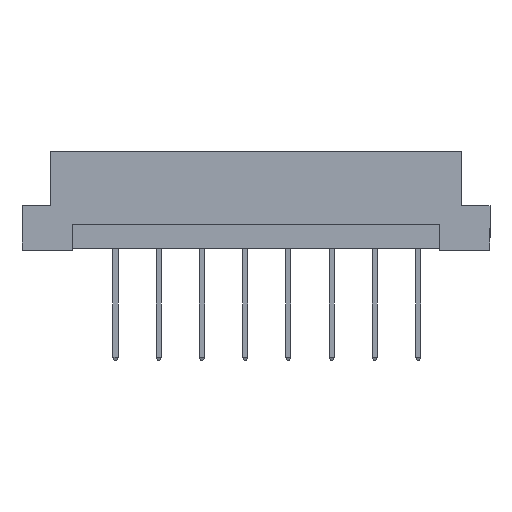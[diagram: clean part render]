
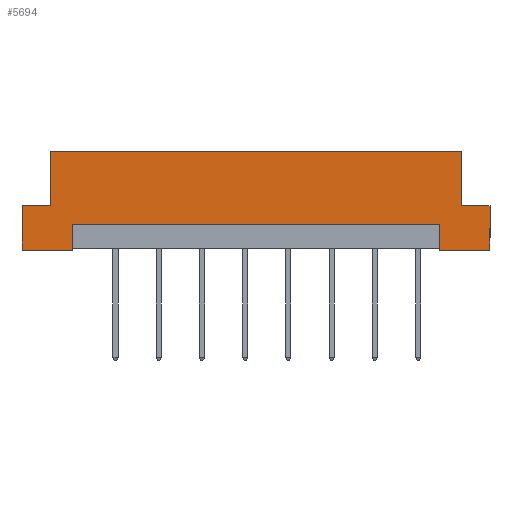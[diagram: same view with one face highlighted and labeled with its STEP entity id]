
A CAD part, front view. The second image highlights one B-rep face of the part: STEP entity #5694.
In plain terms, the highlighted planar face has unit normal (0, -1, 0).
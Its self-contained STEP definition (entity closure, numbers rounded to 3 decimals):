
#69 = ORIENTED_EDGE ( 'NONE', *, *, #2271, .F. ) ;
#78 = VECTOR ( 'NONE', #3230, 1000. ) ;
#87 = VECTOR ( 'NONE', #1869, 1000. ) ;
#91 = VECTOR ( 'NONE', #4804, 1000. ) ;
#100 = CARTESIAN_POINT ( 'NONE',  ( -24.2, -4.3, 5.2 ) ) ;
#203 = EDGE_CURVE ( 'NONE', #1083, #2926, #5327, .T. ) ;
#239 = CARTESIAN_POINT ( 'NONE',  ( 21.6, -4.3, 3. ) ) ;
#248 = ORIENTED_EDGE ( 'NONE', *, *, #5009, .F. ) ;
#266 = DIRECTION ( 'NONE',  ( 1., 0., 0. ) ) ;
#286 = EDGE_CURVE ( 'NONE', #5501, #1397, #1158, .T. ) ;
#299 = DIRECTION ( 'NONE',  ( 0., 0., 1. ) ) ;
#490 = CARTESIAN_POINT ( 'NONE',  ( 27.5, -4.3, 11.6 ) ) ;
#497 = DIRECTION ( 'NONE',  ( 0., 1., 0. ) ) ;
#540 = PLANE ( 'NONE',  #6352 ) ;
#624 = ORIENTED_EDGE ( 'NONE', *, *, #4630, .F. ) ;
#663 = CARTESIAN_POINT ( 'NONE',  ( -21.6, -4.3, 3. ) ) ;
#682 = DIRECTION ( 'NONE',  ( 0., 0., -1. ) ) ;
#715 = CARTESIAN_POINT ( 'NONE',  ( 24.2, -4.3, 11.6 ) ) ;
#798 = VERTEX_POINT ( 'NONE', #4847 ) ;
#1083 = VERTEX_POINT ( 'NONE', #3296 ) ;
#1133 = EDGE_CURVE ( 'NONE', #1083, #5446, #3239, .T. ) ;
#1158 = LINE ( 'NONE', #5298, #78 ) ;
#1261 = LINE ( 'NONE', #5360, #87 ) ;
#1269 = CARTESIAN_POINT ( 'NONE',  ( -24.2, -4.3, 11.6 ) ) ;
#1274 = VECTOR ( 'NONE', #266, 1000. ) ;
#1293 = ORIENTED_EDGE ( 'NONE', *, *, #3089, .T. ) ;
#1309 = LINE ( 'NONE', #3372, #2480 ) ;
#1366 = CARTESIAN_POINT ( 'NONE',  ( 24.2, -4.3, 5.2 ) ) ;
#1397 = VERTEX_POINT ( 'NONE', #5165 ) ;
#1404 = CARTESIAN_POINT ( 'NONE',  ( -21.6, -4.3, 0. ) ) ;
#1427 = ORIENTED_EDGE ( 'NONE', *, *, #4787, .F. ) ;
#1668 = ORIENTED_EDGE ( 'NONE', *, *, #203, .F. ) ;
#1792 = EDGE_CURVE ( 'NONE', #5501, #2680, #5228, .T. ) ;
#1869 = DIRECTION ( 'NONE',  ( 1., 0., 0. ) ) ;
#2163 = DIRECTION ( 'NONE',  ( 0., 0., 1. ) ) ;
#2249 = ORIENTED_EDGE ( 'NONE', *, *, #286, .F. ) ;
#2257 = CARTESIAN_POINT ( 'NONE',  ( 27.5, -4.3, 0. ) ) ;
#2271 = EDGE_CURVE ( 'NONE', #798, #5446, #5050, .T. ) ;
#2384 = ORIENTED_EDGE ( 'NONE', *, *, #1792, .T. ) ;
#2440 = EDGE_CURVE ( 'NONE', #2680, #2926, #5857, .T. ) ;
#2480 = VECTOR ( 'NONE', #299, 1000. ) ;
#2559 = LINE ( 'NONE', #490, #3138 ) ;
#2680 = VERTEX_POINT ( 'NONE', #3476 ) ;
#2686 = VECTOR ( 'NONE', #6101, 1000. ) ;
#2711 = VECTOR ( 'NONE', #5209, 1000. ) ;
#2926 = VERTEX_POINT ( 'NONE', #1404 ) ;
#3089 = EDGE_CURVE ( 'NONE', #6037, #3251, #1309, .T. ) ;
#3138 = VECTOR ( 'NONE', #3602, 1000. ) ;
#3211 = VECTOR ( 'NONE', #3765, 1000. ) ;
#3230 = DIRECTION ( 'NONE',  ( 1., 0., 0. ) ) ;
#3239 = LINE ( 'NONE', #663, #4394 ) ;
#3251 = VERTEX_POINT ( 'NONE', #715 ) ;
#3296 = CARTESIAN_POINT ( 'NONE',  ( -21.6, -4.3, 3. ) ) ;
#3372 = CARTESIAN_POINT ( 'NONE',  ( 24.2, -4.3, 5.2 ) ) ;
#3476 = CARTESIAN_POINT ( 'NONE',  ( -27.5, -4.3, 0. ) ) ;
#3602 = DIRECTION ( 'NONE',  ( 0., 0., -1. ) ) ;
#3636 = LINE ( 'NONE', #4788, #2711 ) ;
#3667 = ORIENTED_EDGE ( 'NONE', *, *, #1133, .T. ) ;
#3765 = DIRECTION ( 'NONE',  ( 1., 0., 0. ) ) ;
#4305 = ORIENTED_EDGE ( 'NONE', *, *, #6326, .T. ) ;
#4394 = VECTOR ( 'NONE', #4792, 1000. ) ;
#4515 = VECTOR ( 'NONE', #682, 1000. ) ;
#4542 = CARTESIAN_POINT ( 'NONE',  ( 21.6, -4.3, 0.2 ) ) ;
#4630 = EDGE_CURVE ( 'NONE', #1397, #4687, #5241, .T. ) ;
#4687 = VERTEX_POINT ( 'NONE', #1269 ) ;
#4723 = CARTESIAN_POINT ( 'NONE',  ( -21.6, -4.3, 0.2 ) ) ;
#4762 = CARTESIAN_POINT ( 'NONE',  ( 27.5, -4.3, 5.2 ) ) ;
#4787 = EDGE_CURVE ( 'NONE', #6281, #5128, #2559, .T. ) ;
#4788 = CARTESIAN_POINT ( 'NONE',  ( 27.5, -4.3, 5.2 ) ) ;
#4792 = DIRECTION ( 'NONE',  ( 1., 0., 0. ) ) ;
#4804 = DIRECTION ( 'NONE',  ( 0., 0., -1. ) ) ;
#4847 = CARTESIAN_POINT ( 'NONE',  ( 21.6, -4.3, 0. ) ) ;
#5009 = EDGE_CURVE ( 'NONE', #6037, #6281, #3636, .T. ) ;
#5050 = LINE ( 'NONE', #4542, #2686 ) ;
#5082 = EDGE_LOOP ( 'NONE', ( #3667, #69, #4305, #1427, #248, #1293, #6299, #624, #2249, #2384, #6522, #1668 ) ) ;
#5128 = VERTEX_POINT ( 'NONE', #5359 ) ;
#5165 = CARTESIAN_POINT ( 'NONE',  ( -24.2, -4.3, 5.2 ) ) ;
#5209 = DIRECTION ( 'NONE',  ( 1., 0., 0. ) ) ;
#5228 = LINE ( 'NONE', #6314, #91 ) ;
#5241 = LINE ( 'NONE', #100, #6385 ) ;
#5298 = CARTESIAN_POINT ( 'NONE',  ( -27.5, -4.3, 5.2 ) ) ;
#5327 = LINE ( 'NONE', #4723, #4515 ) ;
#5359 = CARTESIAN_POINT ( 'NONE',  ( 27.5, -4.3, 0. ) ) ;
#5360 = CARTESIAN_POINT ( 'NONE',  ( 27.5, -4.3, 11.6 ) ) ;
#5446 = VERTEX_POINT ( 'NONE', #239 ) ;
#5501 = VERTEX_POINT ( 'NONE', #5860 ) ;
#5694 = ADVANCED_FACE ( 'NONE', ( #6165 ), #540, .F. ) ;
#5719 = CARTESIAN_POINT ( 'NONE',  ( 27.5, -4.3, 11.6 ) ) ;
#5857 = LINE ( 'NONE', #5957, #1274 ) ;
#5860 = CARTESIAN_POINT ( 'NONE',  ( -27.5, -4.3, 5.2 ) ) ;
#5957 = CARTESIAN_POINT ( 'NONE',  ( 27.5, -4.3, 0. ) ) ;
#6037 = VERTEX_POINT ( 'NONE', #1366 ) ;
#6101 = DIRECTION ( 'NONE',  ( 0., 0., 1. ) ) ;
#6165 = FACE_OUTER_BOUND ( 'NONE', #5082, .T. ) ;
#6198 = DIRECTION ( 'NONE',  ( -1., 0., 0. ) ) ;
#6281 = VERTEX_POINT ( 'NONE', #4762 ) ;
#6299 = ORIENTED_EDGE ( 'NONE', *, *, #6486, .F. ) ;
#6314 = CARTESIAN_POINT ( 'NONE',  ( -27.5, -4.3, 11.6 ) ) ;
#6326 = EDGE_CURVE ( 'NONE', #798, #5128, #6354, .T. ) ;
#6352 = AXIS2_PLACEMENT_3D ( 'NONE', #5719, #497, #6198 ) ;
#6354 = LINE ( 'NONE', #2257, #3211 ) ;
#6385 = VECTOR ( 'NONE', #2163, 1000. ) ;
#6486 = EDGE_CURVE ( 'NONE', #4687, #3251, #1261, .T. ) ;
#6522 = ORIENTED_EDGE ( 'NONE', *, *, #2440, .T. ) ;
